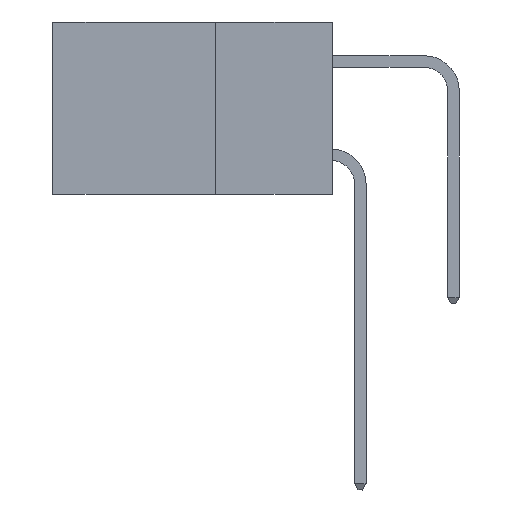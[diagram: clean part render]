
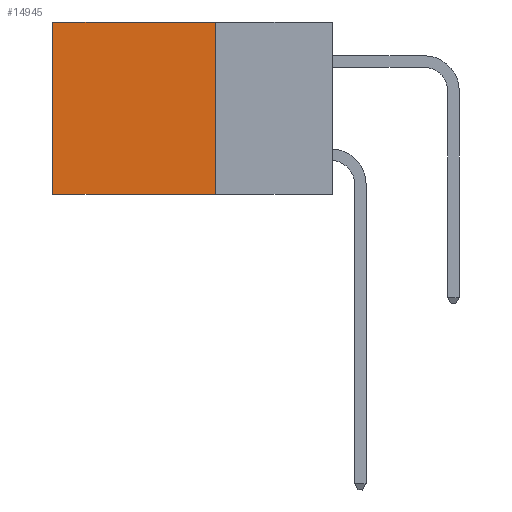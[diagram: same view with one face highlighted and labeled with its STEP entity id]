
A CAD part, left-side view. The second image highlights one B-rep face of the part: STEP entity #14945.
In plain terms, the highlighted planar face has unit normal (-1, 0, 0).
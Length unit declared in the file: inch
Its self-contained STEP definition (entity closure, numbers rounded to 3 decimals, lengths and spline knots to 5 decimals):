
#424 = CARTESIAN_POINT ( 'NONE',  ( 0.2615, 0.25, -0.37 ) ) ;
#1059 = VECTOR ( 'NONE', #6049, 39.37008 ) ;
#2617 = EDGE_CURVE ( 'NONE', #7952, #15875, #27049, .T. ) ;
#2998 = VERTEX_POINT ( 'NONE', #16217 ) ;
#3182 = ORIENTED_EDGE ( 'NONE', *, *, #25124, .T. ) ;
#4808 = VECTOR ( 'NONE', #16917, 39.37008 ) ;
#6049 = DIRECTION ( 'NONE',  ( 0., 1., 0. ) ) ;
#6099 = VECTOR ( 'NONE', #11067, 39.37008 ) ;
#6462 = ORIENTED_EDGE ( 'NONE', *, *, #2617, .T. ) ;
#7333 = ORIENTED_EDGE ( 'NONE', *, *, #22554, .F. ) ;
#7952 = VERTEX_POINT ( 'NONE', #21692 ) ;
#8605 = ORIENTED_EDGE ( 'NONE', *, *, #8895, .F. ) ;
#8895 = EDGE_CURVE ( 'NONE', #2998, #21095, #20623, .T. ) ;
#10689 = CARTESIAN_POINT ( 'NONE',  ( 0.2615, 0.6, -0.37 ) ) ;
#11067 = DIRECTION ( 'NONE',  ( 0., 0., -1. ) ) ;
#12386 = LINE ( 'NONE', #10689, #4808 ) ;
#12458 = DIRECTION ( 'NONE',  ( 0., 1., 0. ) ) ;
#12506 = DIRECTION ( 'NONE',  ( 0., 0., -1. ) ) ;
#14434 = CARTESIAN_POINT ( 'NONE',  ( 0.2615, 0.25, 0. ) ) ;
#14628 = DIRECTION ( 'NONE',  ( 1., 0., 0. ) ) ;
#14945 = ADVANCED_FACE ( 'NONE', ( #16327 ), #25379, .F. ) ;
#15543 = EDGE_LOOP ( 'NONE', ( #3182, #8605, #7333, #6462 ) ) ;
#15875 = VERTEX_POINT ( 'NONE', #17933 ) ;
#16217 = CARTESIAN_POINT ( 'NONE',  ( 0.2615, 0.25, -0.37 ) ) ;
#16327 = FACE_OUTER_BOUND ( 'NONE', #15543, .T. ) ;
#16917 = DIRECTION ( 'NONE',  ( 0., 0., -1. ) ) ;
#17933 = CARTESIAN_POINT ( 'NONE',  ( 0.2615, 0.6, 0. ) ) ;
#18220 = AXIS2_PLACEMENT_3D ( 'NONE', #20995, #14628, #12506 ) ;
#20487 = CARTESIAN_POINT ( 'NONE',  ( 0.2615, 0.25, -0.37 ) ) ;
#20623 = LINE ( 'NONE', #20487, #1059 ) ;
#20995 = CARTESIAN_POINT ( 'NONE',  ( 0.2615, 0.25, -0.37 ) ) ;
#21095 = VERTEX_POINT ( 'NONE', #21552 ) ;
#21552 = CARTESIAN_POINT ( 'NONE',  ( 0.2615, 0.6, -0.37 ) ) ;
#21692 = CARTESIAN_POINT ( 'NONE',  ( 0.2615, 0.25, 0. ) ) ;
#22197 = VECTOR ( 'NONE', #12458, 39.37008 ) ;
#22554 = EDGE_CURVE ( 'NONE', #7952, #2998, #26200, .T. ) ;
#25124 = EDGE_CURVE ( 'NONE', #15875, #21095, #12386, .T. ) ;
#25379 = PLANE ( 'NONE',  #18220 ) ;
#26200 = LINE ( 'NONE', #424, #6099 ) ;
#27049 = LINE ( 'NONE', #14434, #22197 ) ;
